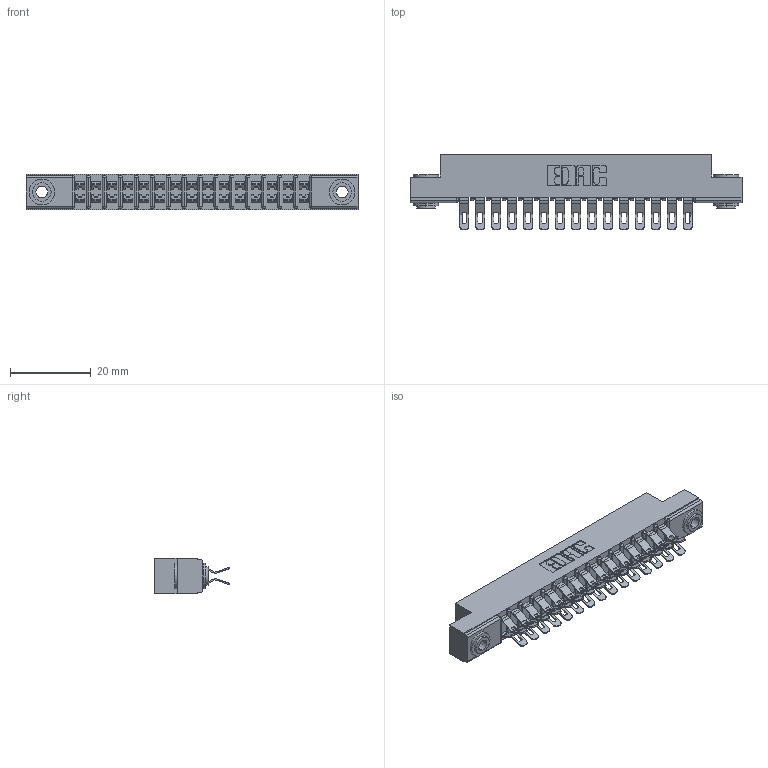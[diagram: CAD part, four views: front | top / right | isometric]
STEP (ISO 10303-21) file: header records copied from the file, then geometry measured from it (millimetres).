
FILE_DESCRIPTION (( 'STEP AP203' ), '1' );
FILE_NAME ('307-030-455-203.STEP', '2020-09-29T09:44:04', ( '' ), ( '' ), 'SwSTEP 2.0', 'SolidWorks 2020', '' );
FILE_SCHEMA (( 'CONFIG_CONTROL_DESIGN' ));
Length unit declared in the file: inch
Products named in the file (4): 307-290-001_555; 307-030-455-203; 345-250-002_345-250-002-102; 307 Part_.156 Dia Mounting Holes
Assembly tree (33 placements, depth 2):
  307-030-455-203
    307 Part_.156 Dia Mounting Holes
    307-290-001_555  x30
    345-250-002_345-250-002-102  x2
Bounding box: 82.45 x 18.75 x 8.71 mm (x, y, z)
Volume: 5484.5 mm3; surface area: 10062.8 mm2
Topology: 33 solids, 33 shells, 2016 faces, 5865 edges, 3822 vertices
Faces by surface type: plane 1114, cylinder 862, sphere 32, cone 8
Entity records: 18270 total; most frequent: CARTESIAN_POINT 2984, DIRECTION 2956, ORIENTED_EDGE 2948, EDGE_CURVE 1474, LINE 1100, VECTOR 1100, VERTEX_POINT 956, AXIS2_PLACEMENT_3D 928
